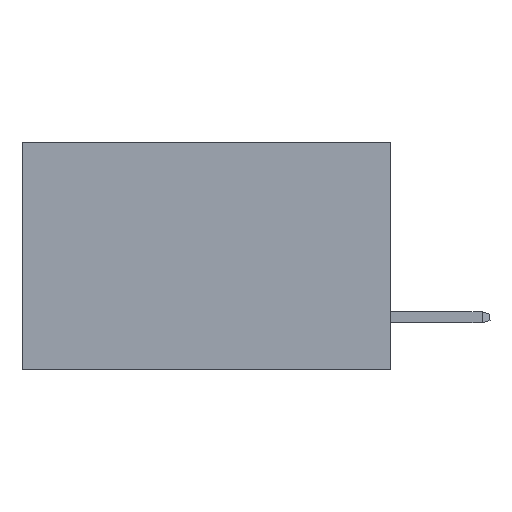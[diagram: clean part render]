
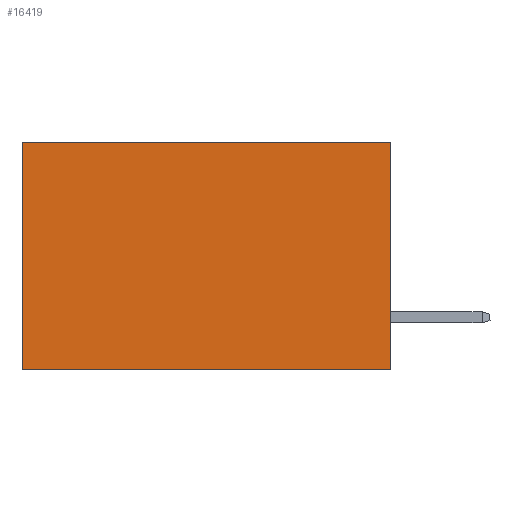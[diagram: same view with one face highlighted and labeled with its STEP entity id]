
A CAD part, left-side view. The second image highlights one B-rep face of the part: STEP entity #16419.
In plain terms, the highlighted planar face has unit normal (-1, 0, 0).
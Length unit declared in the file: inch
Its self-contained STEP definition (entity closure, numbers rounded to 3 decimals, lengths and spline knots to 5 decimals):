
#156 = EDGE_CURVE ( 'NONE', #16370, #23890, #19307, .T. ) ;
#434 = CARTESIAN_POINT ( 'NONE',  ( 0.2875, 0.6, 0. ) ) ;
#817 = DIRECTION ( 'NONE',  ( 0., 0., -1. ) ) ;
#1324 = CARTESIAN_POINT ( 'NONE',  ( 0.2875, 0., -0.37 ) ) ;
#2451 = CARTESIAN_POINT ( 'NONE',  ( 0.2875, 0., 0. ) ) ;
#2986 = PLANE ( 'NONE',  #15004 ) ;
#3242 = CARTESIAN_POINT ( 'NONE',  ( 0.2875, 0.6, -0.37 ) ) ;
#4365 = CARTESIAN_POINT ( 'NONE',  ( 0.2875, 0.6, 0. ) ) ;
#4874 = VECTOR ( 'NONE', #12449, 39.37008 ) ;
#5576 = LINE ( 'NONE', #1324, #4874 ) ;
#6558 = EDGE_CURVE ( 'NONE', #16370, #23316, #26353, .T. ) ;
#6996 = ORIENTED_EDGE ( 'NONE', *, *, #22260, .F. ) ;
#7590 = CARTESIAN_POINT ( 'NONE',  ( 0.2875, 0., 0. ) ) ;
#8333 = ORIENTED_EDGE ( 'NONE', *, *, #156, .T. ) ;
#9464 = CARTESIAN_POINT ( 'NONE',  ( 0.2875, 0., -0.37 ) ) ;
#10121 = ORIENTED_EDGE ( 'NONE', *, *, #6558, .F. ) ;
#10458 = VECTOR ( 'NONE', #21763, 39.37008 ) ;
#11834 = DIRECTION ( 'NONE',  ( 0., 1., 0. ) ) ;
#11905 = DIRECTION ( 'NONE',  ( 1., 0., 0. ) ) ;
#12449 = DIRECTION ( 'NONE',  ( 0., 1., 0. ) ) ;
#14769 = VERTEX_POINT ( 'NONE', #3242 ) ;
#15004 = AXIS2_PLACEMENT_3D ( 'NONE', #18288, #11905, #26924 ) ;
#16370 = VERTEX_POINT ( 'NONE', #2451 ) ;
#16419 = ADVANCED_FACE ( 'NONE', ( #24446 ), #2986, .F. ) ;
#16875 = LINE ( 'NONE', #4365, #10458 ) ;
#18219 = CARTESIAN_POINT ( 'NONE',  ( 0.2875, 0., 0. ) ) ;
#18288 = CARTESIAN_POINT ( 'NONE',  ( 0.2875, 0., 0. ) ) ;
#19307 = LINE ( 'NONE', #18219, #25686 ) ;
#20609 = VECTOR ( 'NONE', #817, 39.37008 ) ;
#20650 = EDGE_CURVE ( 'NONE', #23890, #14769, #16875, .T. ) ;
#21763 = DIRECTION ( 'NONE',  ( 0., 0., -1. ) ) ;
#22260 = EDGE_CURVE ( 'NONE', #23316, #14769, #5576, .T. ) ;
#23316 = VERTEX_POINT ( 'NONE', #9464 ) ;
#23387 = EDGE_LOOP ( 'NONE', ( #27021, #6996, #10121, #8333 ) ) ;
#23890 = VERTEX_POINT ( 'NONE', #434 ) ;
#24446 = FACE_OUTER_BOUND ( 'NONE', #23387, .T. ) ;
#25686 = VECTOR ( 'NONE', #11834, 39.37008 ) ;
#26353 = LINE ( 'NONE', #7590, #20609 ) ;
#26924 = DIRECTION ( 'NONE',  ( 0., 0., -1. ) ) ;
#27021 = ORIENTED_EDGE ( 'NONE', *, *, #20650, .T. ) ;
